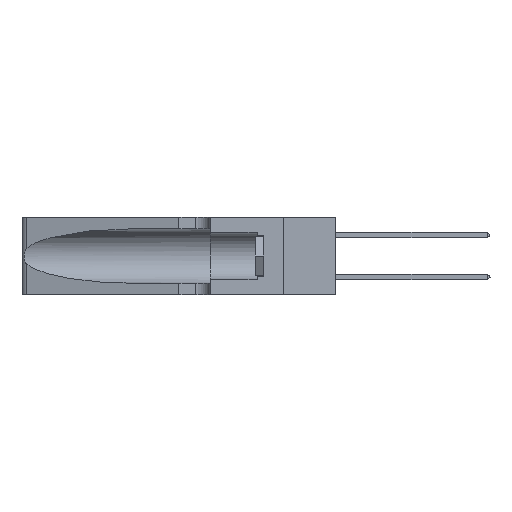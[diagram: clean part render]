
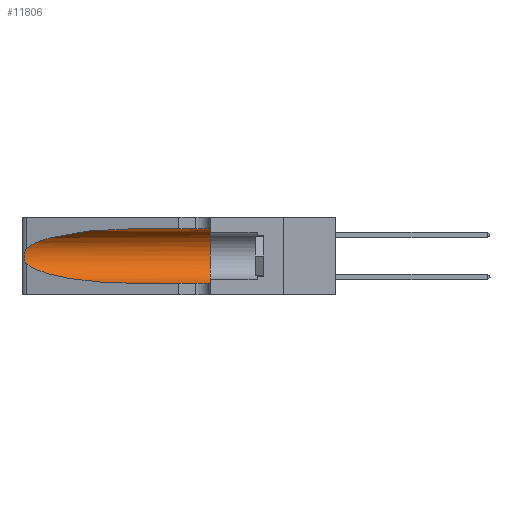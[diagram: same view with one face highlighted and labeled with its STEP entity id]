
A CAD part, left-side view. The second image highlights one B-rep face of the part: STEP entity #11806.
In plain terms, the highlighted cylindrical face has radius 3.308 mm (diameter 6.617 mm), a partial arc.
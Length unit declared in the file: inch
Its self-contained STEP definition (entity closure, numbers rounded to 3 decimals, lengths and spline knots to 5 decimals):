
#221 =( BOUNDED_CURVE ( )  B_SPLINE_CURVE ( 3, ( #5227, #33182, #3306, #13263 ),
 .UNSPECIFIED., .F., .T. ) 
 B_SPLINE_CURVE_WITH_KNOTS ( ( 4, 4 ),
 ( 3.44316, 4.71239 ),
 .UNSPECIFIED. ) 
 CURVE ( )  GEOMETRIC_REPRESENTATION_ITEM ( )  RATIONAL_B_SPLINE_CURVE ( ( 1., 0.87, 0.87, 1. ) ) 
 REPRESENTATION_ITEM ( '' )  );
#648 = FACE_OUTER_BOUND ( 'NONE', #29316, .T. ) ;
#1115 = DIRECTION ( 'NONE',  ( 0., -1., 0. ) ) ;
#1198 = VERTEX_POINT ( 'NONE', #23196 ) ;
#1459 = ORIENTED_EDGE ( 'NONE', *, *, #16659, .F. ) ;
#1472 = CARTESIAN_POINT ( 'NONE',  ( 0.26018, 1.23835, 0.19895 ) ) ;
#3106 = B_SPLINE_CURVE_WITH_KNOTS ( 'NONE', 3,
 ( #27351, #16700, #6957, #11981, #26999, #1472, #17189, #11631, #19393, #21972, #19626, #6594, #24518, #24870 ),
 .UNSPECIFIED., .F., .F.,
 ( 4, 2, 2, 2, 2, 2, 4 ),
 ( 0., 0.00027, 0.00053, 0.00107, 0.0016, 0.00187, 0.00214 ),
 .UNSPECIFIED. ) ;
#3306 = CARTESIAN_POINT ( 'NONE',  ( 0.18966, 0.96281, 0.05475 ) ) ;
#5227 = CARTESIAN_POINT ( 'NONE',  ( 0.25487, 1.22718, 0.14631 ) ) ;
#5628 = AXIS2_PLACEMENT_3D ( 'NONE', #20997, #21439, #8442 ) ;
#6226 = ORIENTED_EDGE ( 'NONE', *, *, #22456, .T. ) ;
#6488 = EDGE_CURVE ( 'NONE', #7191, #1198, #22774, .T. ) ;
#6594 = CARTESIAN_POINT ( 'NONE',  ( 0.25639, 1.23186, 0.15144 ) ) ;
#6915 = CARTESIAN_POINT ( 'NONE',  ( 0.1305, 0.35, 0.185 ) ) ;
#6957 = CARTESIAN_POINT ( 'NONE',  ( 0.25639, 1.23184, 0.21858 ) ) ;
#7191 = VERTEX_POINT ( 'NONE', #22248 ) ;
#8112 = AXIS2_PLACEMENT_3D ( 'NONE', #6915, #29903, #17145 ) ;
#8442 = DIRECTION ( 'NONE',  ( 0., 0., -1. ) ) ;
#9905 = LINE ( 'NONE', #30698, #28344 ) ;
#10451 = CARTESIAN_POINT ( 'NONE',  ( 0.25487, 1.22718, 0.22369 ) ) ;
#10769 = CARTESIAN_POINT ( 'NONE',  ( 0.1305, 0.72297, 0.31525 ) ) ;
#11475 = VERTEX_POINT ( 'NONE', #14066 ) ;
#11631 = CARTESIAN_POINT ( 'NONE',  ( 0.26075, 1.23896, 0.178 ) ) ;
#11806 = ADVANCED_FACE ( 'NONE', ( #648 ), #27588, .F. ) ;
#11981 = CARTESIAN_POINT ( 'NONE',  ( 0.25787, 1.23484, 0.2124 ) ) ;
#12632 = EDGE_CURVE ( 'NONE', #28743, #29445, #9905, .T. ) ;
#13263 = CARTESIAN_POINT ( 'NONE',  ( 0.1305, 0.72297, 0.05475 ) ) ;
#13650 = CARTESIAN_POINT ( 'NONE',  ( 0.2373, 1.15595, 0.28018 ) ) ;
#14066 = CARTESIAN_POINT ( 'NONE',  ( 0.25487, 1.22718, 0.14631 ) ) ;
#15844 = ORIENTED_EDGE ( 'NONE', *, *, #24393, .T. ) ;
#16659 = EDGE_CURVE ( 'NONE', #1198, #29445, #21355, .T. ) ;
#16700 = CARTESIAN_POINT ( 'NONE',  ( 0.25555, 1.22994, 0.2215 ) ) ;
#17145 = DIRECTION ( 'NONE',  ( 0., 0., 1. ) ) ;
#17189 = CARTESIAN_POINT ( 'NONE',  ( 0.26075, 1.23896, 0.19203 ) ) ;
#18827 = CARTESIAN_POINT ( 'NONE',  ( 0.25487, 1.22718, 0.22369 ) ) ;
#19393 = CARTESIAN_POINT ( 'NONE',  ( 0.26017, 1.23833, 0.17102 ) ) ;
#19626 = CARTESIAN_POINT ( 'NONE',  ( 0.25789, 1.23486, 0.15765 ) ) ;
#20716 = CARTESIAN_POINT ( 'NONE',  ( 0.1305, 0.35, 0.05475 ) ) ;
#20997 = CARTESIAN_POINT ( 'NONE',  ( 0.1305, 1.61858, 0.185 ) ) ;
#21355 = CIRCLE ( 'NONE', #8112, 0.13025 ) ;
#21439 = DIRECTION ( 'NONE',  ( 0., -1., 0. ) ) ;
#21972 = CARTESIAN_POINT ( 'NONE',  ( 0.25856, 1.23593, 0.16098 ) ) ;
#22248 = CARTESIAN_POINT ( 'NONE',  ( 0.1305, 0.72297, 0.31525 ) ) ;
#22456 = EDGE_CURVE ( 'NONE', #7191, #25498, #24458, .T. ) ;
#22495 = ORIENTED_EDGE ( 'NONE', *, *, #12632, .T. ) ;
#22774 = LINE ( 'NONE', #24423, #28009 ) ;
#22839 = DIRECTION ( 'NONE',  ( 0., -1., 0. ) ) ;
#23196 = CARTESIAN_POINT ( 'NONE',  ( 0.1305, 0.35, 0.31525 ) ) ;
#23864 = ORIENTED_EDGE ( 'NONE', *, *, #6488, .F. ) ;
#24393 = EDGE_CURVE ( 'NONE', #11475, #28743, #221, .T. ) ;
#24423 = CARTESIAN_POINT ( 'NONE',  ( 0.1305, 1.61858, 0.31525 ) ) ;
#24458 =( BOUNDED_CURVE ( )  B_SPLINE_CURVE ( 3, ( #10769, #31204, #13650, #18827 ),
 .UNSPECIFIED., .F., .T. ) 
 B_SPLINE_CURVE_WITH_KNOTS ( ( 4, 4 ),
 ( 1.5708, 2.84003 ),
 .UNSPECIFIED. ) 
 CURVE ( )  GEOMETRIC_REPRESENTATION_ITEM ( )  RATIONAL_B_SPLINE_CURVE ( ( 1., 0.87, 0.87, 1. ) ) 
 REPRESENTATION_ITEM ( '' )  );
#24518 = CARTESIAN_POINT ( 'NONE',  ( 0.25555, 1.22993, 0.14849 ) ) ;
#24870 = CARTESIAN_POINT ( 'NONE',  ( 0.25487, 1.22718, 0.14631 ) ) ;
#25498 = VERTEX_POINT ( 'NONE', #10451 ) ;
#25812 = ORIENTED_EDGE ( 'NONE', *, *, #29176, .T. ) ;
#26999 = CARTESIAN_POINT ( 'NONE',  ( 0.25854, 1.2359, 0.20912 ) ) ;
#27351 = CARTESIAN_POINT ( 'NONE',  ( 0.25487, 1.22718, 0.22369 ) ) ;
#27588 = CYLINDRICAL_SURFACE ( 'NONE', #5628, 0.13025 ) ;
#28009 = VECTOR ( 'NONE', #1115, 39.37008 ) ;
#28344 = VECTOR ( 'NONE', #22839, 39.37008 ) ;
#28743 = VERTEX_POINT ( 'NONE', #30570 ) ;
#29176 = EDGE_CURVE ( 'NONE', #25498, #11475, #3106, .T. ) ;
#29316 = EDGE_LOOP ( 'NONE', ( #6226, #25812, #15844, #22495, #1459, #23864 ) ) ;
#29445 = VERTEX_POINT ( 'NONE', #20716 ) ;
#29903 = DIRECTION ( 'NONE',  ( 0., 1., 0. ) ) ;
#30570 = CARTESIAN_POINT ( 'NONE',  ( 0.1305, 0.72297, 0.05475 ) ) ;
#30698 = CARTESIAN_POINT ( 'NONE',  ( 0.1305, 1.61858, 0.05475 ) ) ;
#31204 = CARTESIAN_POINT ( 'NONE',  ( 0.18966, 0.96281, 0.31525 ) ) ;
#33182 = CARTESIAN_POINT ( 'NONE',  ( 0.2373, 1.15595, 0.08982 ) ) ;
